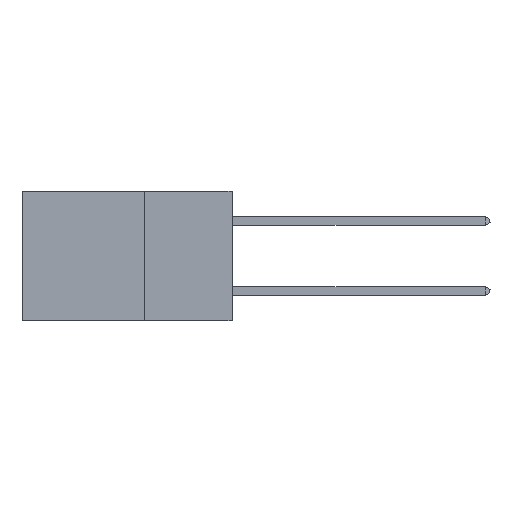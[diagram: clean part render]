
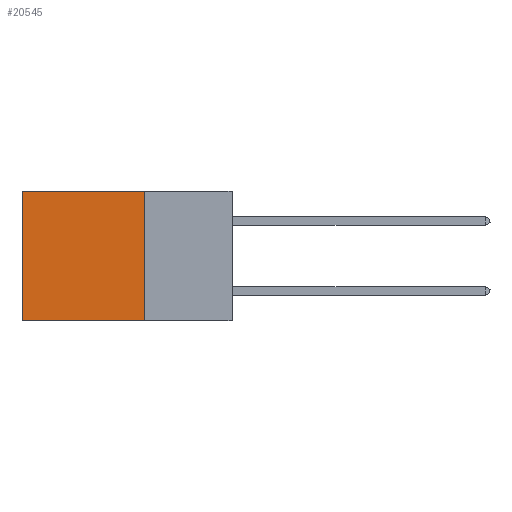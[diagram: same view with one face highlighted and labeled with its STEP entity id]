
A CAD part, left-side view. The second image highlights one B-rep face of the part: STEP entity #20545.
In plain terms, the highlighted planar face has unit normal (-1, 0, 0).
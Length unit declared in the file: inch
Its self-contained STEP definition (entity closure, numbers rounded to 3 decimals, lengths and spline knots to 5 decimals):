
#343 = ORIENTED_EDGE ( 'NONE', *, *, #13339, .F. ) ;
#707 = DIRECTION ( 'NONE',  ( 0., 0., -1. ) ) ;
#918 = PLANE ( 'NONE',  #6795 ) ;
#1014 = EDGE_LOOP ( 'NONE', ( #5353, #343, #11663, #6950 ) ) ;
#1039 = CARTESIAN_POINT ( 'NONE',  ( 0.2875, 0.25, 0. ) ) ;
#1669 = EDGE_CURVE ( 'NONE', #15139, #19986, #13981, .T. ) ;
#2746 = DIRECTION ( 'NONE',  ( 1., 0., 0. ) ) ;
#2872 = DIRECTION ( 'NONE',  ( 0., 1., 0. ) ) ;
#3178 = VECTOR ( 'NONE', #15178, 39.37008 ) ;
#4703 = EDGE_CURVE ( 'NONE', #4820, #16812, #20372, .T. ) ;
#4820 = VERTEX_POINT ( 'NONE', #16031 ) ;
#5353 = ORIENTED_EDGE ( 'NONE', *, *, #1669, .T. ) ;
#5457 = CARTESIAN_POINT ( 'NONE',  ( 0.2875, 0.25, 0. ) ) ;
#6795 = AXIS2_PLACEMENT_3D ( 'NONE', #11470, #2746, #14891 ) ;
#6950 = ORIENTED_EDGE ( 'NONE', *, *, #13935, .T. ) ;
#8833 = VECTOR ( 'NONE', #707, 39.37008 ) ;
#9359 = FACE_OUTER_BOUND ( 'NONE', #1014, .T. ) ;
#10251 = VECTOR ( 'NONE', #2872, 39.37008 ) ;
#11470 = CARTESIAN_POINT ( 'NONE',  ( 0.2875, 0.25, 0. ) ) ;
#11663 = ORIENTED_EDGE ( 'NONE', *, *, #4703, .F. ) ;
#12354 = CARTESIAN_POINT ( 'NONE',  ( 0.2875, 0.25, -0.37 ) ) ;
#13339 = EDGE_CURVE ( 'NONE', #16812, #19986, #16890, .T. ) ;
#13496 = CARTESIAN_POINT ( 'NONE',  ( 0.2875, 0.25, -0.37 ) ) ;
#13935 = EDGE_CURVE ( 'NONE', #4820, #15139, #19225, .T. ) ;
#13981 = LINE ( 'NONE', #17971, #8833 ) ;
#14891 = DIRECTION ( 'NONE',  ( 0., 0., -1. ) ) ;
#14994 = CARTESIAN_POINT ( 'NONE',  ( 0.2875, 0.6, -0.37 ) ) ;
#15139 = VERTEX_POINT ( 'NONE', #21568 ) ;
#15178 = DIRECTION ( 'NONE',  ( 0., 1., 0. ) ) ;
#16031 = CARTESIAN_POINT ( 'NONE',  ( 0.2875, 0.25, 0. ) ) ;
#16812 = VERTEX_POINT ( 'NONE', #12354 ) ;
#16890 = LINE ( 'NONE', #13496, #3178 ) ;
#17424 = DIRECTION ( 'NONE',  ( 0., 0., -1. ) ) ;
#17971 = CARTESIAN_POINT ( 'NONE',  ( 0.2875, 0.6, 0. ) ) ;
#19225 = LINE ( 'NONE', #1039, #10251 ) ;
#19986 = VERTEX_POINT ( 'NONE', #14994 ) ;
#20372 = LINE ( 'NONE', #5457, #21387 ) ;
#20545 = ADVANCED_FACE ( 'NONE', ( #9359 ), #918, .F. ) ;
#21387 = VECTOR ( 'NONE', #17424, 39.37008 ) ;
#21568 = CARTESIAN_POINT ( 'NONE',  ( 0.2875, 0.6, 0. ) ) ;
